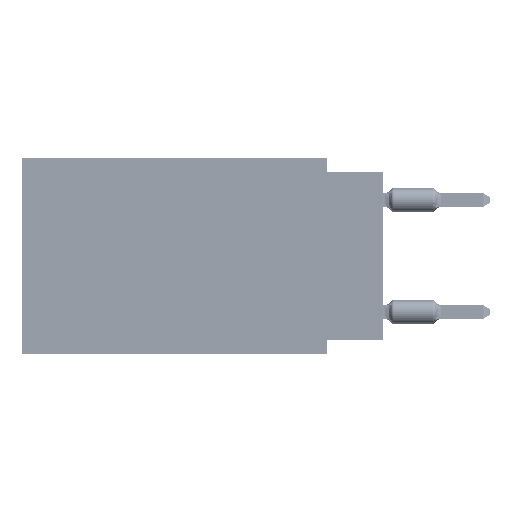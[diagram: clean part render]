
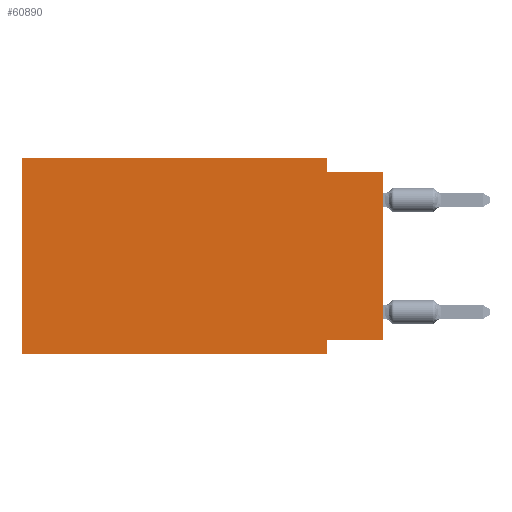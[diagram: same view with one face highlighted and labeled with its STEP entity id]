
A CAD part, left-side view. The second image highlights one B-rep face of the part: STEP entity #60890.
In plain terms, the highlighted planar face has unit normal (-1, 0, 0).
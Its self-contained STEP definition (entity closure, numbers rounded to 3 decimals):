
#1607 = EDGE_CURVE ( 'NONE', #59687, #7804, #59592, .T. ) ;
#1791 = DIRECTION ( 'NONE',  ( 0., 0., 1. ) ) ;
#2055 = LINE ( 'NONE', #60474, #65044 ) ;
#2597 = VERTEX_POINT ( 'NONE', #61317 ) ;
#2813 = CARTESIAN_POINT ( 'NONE',  ( 0., 0., -0.635 ) ) ;
#3127 = EDGE_CURVE ( 'NONE', #60784, #50430, #52275, .T. ) ;
#5571 = VERTEX_POINT ( 'NONE', #46565 ) ;
#5952 = AXIS2_PLACEMENT_3D ( 'NONE', #44236, #65214, #48375 ) ;
#6421 = EDGE_CURVE ( 'NONE', #5571, #12546, #38494, .T. ) ;
#6605 = VECTOR ( 'NONE', #32673, 1000. ) ;
#7350 = CARTESIAN_POINT ( 'NONE',  ( 0., 0., -8.255 ) ) ;
#7804 = VERTEX_POINT ( 'NONE', #41216 ) ;
#9668 = CARTESIAN_POINT ( 'NONE',  ( 0., 2.54, 0. ) ) ;
#12546 = VERTEX_POINT ( 'NONE', #59459 ) ;
#12630 = PLANE ( 'NONE',  #5952 ) ;
#14488 = DIRECTION ( 'NONE',  ( 0., -1., 0. ) ) ;
#16140 = EDGE_LOOP ( 'NONE', ( #61706, #16312, #19106, #34838, #24358, #22947, #41753, #30700 ) ) ;
#16312 = ORIENTED_EDGE ( 'NONE', *, *, #3127, .F. ) ;
#17766 = CARTESIAN_POINT ( 'NONE',  ( 0., 0., -8.255 ) ) ;
#18000 = DIRECTION ( 'NONE',  ( 0., 1., 0. ) ) ;
#18850 = LINE ( 'NONE', #24710, #24415 ) ;
#19106 = ORIENTED_EDGE ( 'NONE', *, *, #40224, .F. ) ;
#21001 = CARTESIAN_POINT ( 'NONE',  ( 0., 0., -0.635 ) ) ;
#22947 = ORIENTED_EDGE ( 'NONE', *, *, #6421, .T. ) ;
#24358 = ORIENTED_EDGE ( 'NONE', *, *, #49774, .F. ) ;
#24415 = VECTOR ( 'NONE', #54944, 1000. ) ;
#24710 = CARTESIAN_POINT ( 'NONE',  ( 0., 2.54, -8.89 ) ) ;
#26061 = EDGE_CURVE ( 'NONE', #59687, #50430, #60218, .T. ) ;
#27427 = FACE_OUTER_BOUND ( 'NONE', #16140, .T. ) ;
#27762 = VECTOR ( 'NONE', #14488, 1000. ) ;
#28604 = CARTESIAN_POINT ( 'NONE',  ( 0., 0., 0. ) ) ;
#29951 = VECTOR ( 'NONE', #1791, 1000. ) ;
#30700 = ORIENTED_EDGE ( 'NONE', *, *, #1607, .F. ) ;
#30891 = CARTESIAN_POINT ( 'NONE',  ( 0., 2.54, -0.635 ) ) ;
#31683 = EDGE_CURVE ( 'NONE', #7804, #12546, #18850, .T. ) ;
#32673 = DIRECTION ( 'NONE',  ( 0., -1., 0. ) ) ;
#34838 = ORIENTED_EDGE ( 'NONE', *, *, #50493, .F. ) ;
#35111 = LINE ( 'NONE', #61574, #27762 ) ;
#37404 = CARTESIAN_POINT ( 'NONE',  ( 0., 2.54, 0. ) ) ;
#38494 = LINE ( 'NONE', #49479, #60533 ) ;
#40224 = EDGE_CURVE ( 'NONE', #43931, #60784, #43575, .T. ) ;
#41216 = CARTESIAN_POINT ( 'NONE',  ( 0., 2.54, -8.255 ) ) ;
#41753 = ORIENTED_EDGE ( 'NONE', *, *, #31683, .F. ) ;
#43257 = VECTOR ( 'NONE', #64206, 1000. ) ;
#43575 = LINE ( 'NONE', #37404, #43257 ) ;
#43931 = VERTEX_POINT ( 'NONE', #9668 ) ;
#44236 = CARTESIAN_POINT ( 'NONE',  ( 0., 16.383, 0. ) ) ;
#46565 = CARTESIAN_POINT ( 'NONE',  ( 0., 16.383, -8.89 ) ) ;
#48375 = DIRECTION ( 'NONE',  ( 0., 0., -1. ) ) ;
#49479 = CARTESIAN_POINT ( 'NONE',  ( 0., 16.383, -8.89 ) ) ;
#49774 = EDGE_CURVE ( 'NONE', #5571, #2597, #2055, .T. ) ;
#50430 = VERTEX_POINT ( 'NONE', #2813 ) ;
#50493 = EDGE_CURVE ( 'NONE', #2597, #43931, #35111, .T. ) ;
#52275 = LINE ( 'NONE', #21001, #6605 ) ;
#54944 = DIRECTION ( 'NONE',  ( 0., 0., -1. ) ) ;
#55826 = VECTOR ( 'NONE', #18000, 1000. ) ;
#59123 = DIRECTION ( 'NONE',  ( 0., -1., 0. ) ) ;
#59459 = CARTESIAN_POINT ( 'NONE',  ( 0., 2.54, -8.89 ) ) ;
#59592 = LINE ( 'NONE', #7350, #55826 ) ;
#59687 = VERTEX_POINT ( 'NONE', #17766 ) ;
#60218 = LINE ( 'NONE', #28604, #29951 ) ;
#60474 = CARTESIAN_POINT ( 'NONE',  ( 0., 16.383, 0. ) ) ;
#60533 = VECTOR ( 'NONE', #59123, 1000. ) ;
#60784 = VERTEX_POINT ( 'NONE', #30891 ) ;
#60890 = ADVANCED_FACE ( 'NONE', ( #27427 ), #12630, .F. ) ;
#61317 = CARTESIAN_POINT ( 'NONE',  ( 0., 16.383, 0. ) ) ;
#61574 = CARTESIAN_POINT ( 'NONE',  ( 0., 16.383, 0. ) ) ;
#61706 = ORIENTED_EDGE ( 'NONE', *, *, #26061, .T. ) ;
#64206 = DIRECTION ( 'NONE',  ( 0., 0., -1. ) ) ;
#65044 = VECTOR ( 'NONE', #65633, 1000. ) ;
#65214 = DIRECTION ( 'NONE',  ( 1., 0., 0. ) ) ;
#65633 = DIRECTION ( 'NONE',  ( 0., 0., 1. ) ) ;
